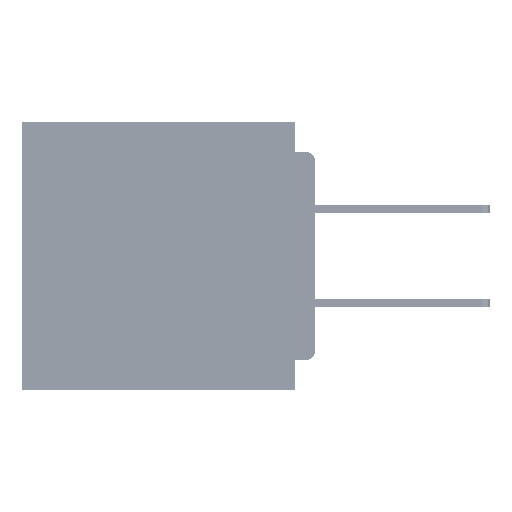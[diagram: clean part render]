
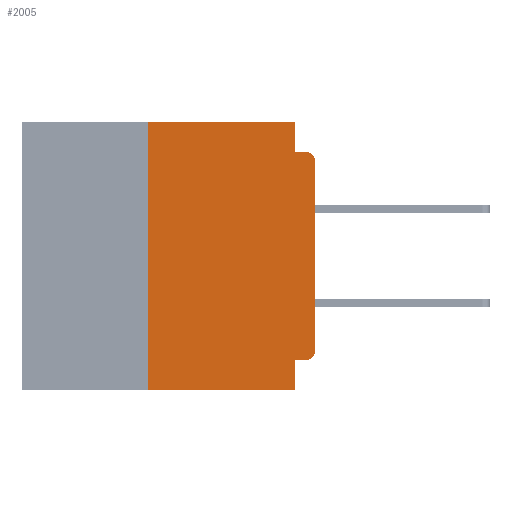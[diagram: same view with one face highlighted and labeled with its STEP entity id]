
A CAD part, left-side view. The second image highlights one B-rep face of the part: STEP entity #2005.
In plain terms, the highlighted planar face has unit normal (-1, 0, 0).
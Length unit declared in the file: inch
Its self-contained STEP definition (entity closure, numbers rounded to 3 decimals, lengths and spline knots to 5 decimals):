
#30 = CARTESIAN_POINT ( 'NONE',  ( 0., 0.015, -0.06 ) ) ;
#140 = CIRCLE ( 'NONE', #52685, 0.015 ) ;
#1220 = DIRECTION ( 'NONE',  ( 0., 0., -1. ) ) ;
#1701 = EDGE_CURVE ( 'NONE', #68793, #38437, #60307, .T. ) ;
#1865 = CARTESIAN_POINT ( 'NONE',  ( 0., 0., -0.355 ) ) ;
#2005 = ADVANCED_FACE ( 'NONE', ( #68743 ), #63641, .F. ) ;
#3260 = LINE ( 'NONE', #44573, #57825 ) ;
#3632 = DIRECTION ( 'NONE',  ( 0., -1., 0. ) ) ;
#3877 = DIRECTION ( 'NONE',  ( 1., 0., 0. ) ) ;
#5523 = DIRECTION ( 'NONE',  ( 0., 0., -1. ) ) ;
#8135 = ORIENTED_EDGE ( 'NONE', *, *, #63493, .F. ) ;
#8529 = CARTESIAN_POINT ( 'NONE',  ( 0., 0.25, 0. ) ) ;
#9770 = CARTESIAN_POINT ( 'NONE',  ( 0., 0., -0.06 ) ) ;
#9825 = EDGE_CURVE ( 'NONE', #35159, #38437, #140, .T. ) ;
#10263 = VECTOR ( 'NONE', #44187, 39.37008 ) ;
#11371 = EDGE_LOOP ( 'NONE', ( #38533, #64787, #14103, #8135, #43677, #55201, #49261, #44193, #22524, #68256 ) ) ;
#11526 = CARTESIAN_POINT ( 'NONE',  ( 0., 0.031, -0.4 ) ) ;
#11947 = CARTESIAN_POINT ( 'NONE',  ( 0., 0.015, -0.355 ) ) ;
#13939 = VERTEX_POINT ( 'NONE', #8529 ) ;
#14103 = ORIENTED_EDGE ( 'NONE', *, *, #1701, .F. ) ;
#14542 = CARTESIAN_POINT ( 'NONE',  ( 0., 0.015, -0.34 ) ) ;
#16352 = AXIS2_PLACEMENT_3D ( 'NONE', #69118, #3877, #41982 ) ;
#16402 = DIRECTION ( 'NONE',  ( 0., -1., 0. ) ) ;
#17118 = CARTESIAN_POINT ( 'NONE',  ( 0., 0., -0.045 ) ) ;
#19392 = CARTESIAN_POINT ( 'NONE',  ( 0., 0.437, 0. ) ) ;
#20060 = DIRECTION ( 'NONE',  ( 0., 0., -1. ) ) ;
#22524 = ORIENTED_EDGE ( 'NONE', *, *, #31351, .F. ) ;
#23644 = LINE ( 'NONE', #1865, #65409 ) ;
#23851 = CARTESIAN_POINT ( 'NONE',  ( 0., 0.031, -0.4 ) ) ;
#24432 = VECTOR ( 'NONE', #60836, 39.37008 ) ;
#24821 = VERTEX_POINT ( 'NONE', #49899 ) ;
#25024 = VERTEX_POINT ( 'NONE', #57285 ) ;
#25951 = LINE ( 'NONE', #53946, #69437 ) ;
#26148 = LINE ( 'NONE', #49865, #24432 ) ;
#29723 = AXIS2_PLACEMENT_3D ( 'NONE', #14542, #52686, #20060 ) ;
#31351 = EDGE_CURVE ( 'NONE', #34814, #38468, #23644, .T. ) ;
#32025 = EDGE_CURVE ( 'NONE', #13939, #33624, #53392, .T. ) ;
#32485 = CARTESIAN_POINT ( 'NONE',  ( 0., 0.015, -0.045 ) ) ;
#33624 = VERTEX_POINT ( 'NONE', #48514 ) ;
#34538 = VECTOR ( 'NONE', #3632, 39.37008 ) ;
#34814 = VERTEX_POINT ( 'NONE', #11947 ) ;
#35159 = VERTEX_POINT ( 'NONE', #9770 ) ;
#35412 = CIRCLE ( 'NONE', #29723, 0.015 ) ;
#38163 = DIRECTION ( 'NONE',  ( -1., 0., 0. ) ) ;
#38437 = VERTEX_POINT ( 'NONE', #32485 ) ;
#38468 = VERTEX_POINT ( 'NONE', #54626 ) ;
#38533 = ORIENTED_EDGE ( 'NONE', *, *, #42005, .T. ) ;
#38687 = VERTEX_POINT ( 'NONE', #23851 ) ;
#39967 = DIRECTION ( 'NONE',  ( 0., 1., 0. ) ) ;
#41736 = CARTESIAN_POINT ( 'NONE',  ( 0., 0.437, -0.4 ) ) ;
#41982 = DIRECTION ( 'NONE',  ( 0., 0., -1. ) ) ;
#42005 = EDGE_CURVE ( 'NONE', #24821, #35159, #25951, .T. ) ;
#43677 = ORIENTED_EDGE ( 'NONE', *, *, #32025, .F. ) ;
#44187 = DIRECTION ( 'NONE',  ( 0., 0., -1. ) ) ;
#44193 = ORIENTED_EDGE ( 'NONE', *, *, #54124, .F. ) ;
#44573 = CARTESIAN_POINT ( 'NONE',  ( 0., 0.031, 0. ) ) ;
#46625 = EDGE_CURVE ( 'NONE', #25024, #38687, #49043, .T. ) ;
#47514 = VECTOR ( 'NONE', #16402, 39.37008 ) ;
#48514 = CARTESIAN_POINT ( 'NONE',  ( 0., 0.031, 0. ) ) ;
#49043 = LINE ( 'NONE', #41736, #34538 ) ;
#49261 = ORIENTED_EDGE ( 'NONE', *, *, #46625, .T. ) ;
#49865 = CARTESIAN_POINT ( 'NONE',  ( 0., 0.25, -0.4 ) ) ;
#49899 = CARTESIAN_POINT ( 'NONE',  ( 0., 0., -0.34 ) ) ;
#52056 = LINE ( 'NONE', #11526, #10263 ) ;
#52685 = AXIS2_PLACEMENT_3D ( 'NONE', #30, #38163, #5523 ) ;
#52686 = DIRECTION ( 'NONE',  ( -1., 0., 0. ) ) ;
#53392 = LINE ( 'NONE', #19392, #66164 ) ;
#53946 = CARTESIAN_POINT ( 'NONE',  ( 0., 0., 0. ) ) ;
#54124 = EDGE_CURVE ( 'NONE', #38468, #38687, #52056, .T. ) ;
#54626 = CARTESIAN_POINT ( 'NONE',  ( 0., 0.031, -0.355 ) ) ;
#55201 = ORIENTED_EDGE ( 'NONE', *, *, #57010, .F. ) ;
#57010 = EDGE_CURVE ( 'NONE', #25024, #13939, #26148, .T. ) ;
#57285 = CARTESIAN_POINT ( 'NONE',  ( 0., 0.25, -0.4 ) ) ;
#57559 = DIRECTION ( 'NONE',  ( 0., -1., 0. ) ) ;
#57825 = VECTOR ( 'NONE', #1220, 39.37008 ) ;
#60307 = LINE ( 'NONE', #17118, #47514 ) ;
#60663 = CARTESIAN_POINT ( 'NONE',  ( 0., 0.031, -0.045 ) ) ;
#60836 = DIRECTION ( 'NONE',  ( 0., 0., 1. ) ) ;
#63493 = EDGE_CURVE ( 'NONE', #33624, #68793, #3260, .T. ) ;
#63641 = PLANE ( 'NONE',  #16352 ) ;
#64787 = ORIENTED_EDGE ( 'NONE', *, *, #9825, .T. ) ;
#65409 = VECTOR ( 'NONE', #39967, 39.37008 ) ;
#66164 = VECTOR ( 'NONE', #57559, 39.37008 ) ;
#68256 = ORIENTED_EDGE ( 'NONE', *, *, #68318, .T. ) ;
#68318 = EDGE_CURVE ( 'NONE', #34814, #24821, #35412, .T. ) ;
#68743 = FACE_OUTER_BOUND ( 'NONE', #11371, .T. ) ;
#68793 = VERTEX_POINT ( 'NONE', #60663 ) ;
#69118 = CARTESIAN_POINT ( 'NONE',  ( 0., 0.437, 0. ) ) ;
#69437 = VECTOR ( 'NONE', #70154, 39.37008 ) ;
#70154 = DIRECTION ( 'NONE',  ( 0., 0., 1. ) ) ;
